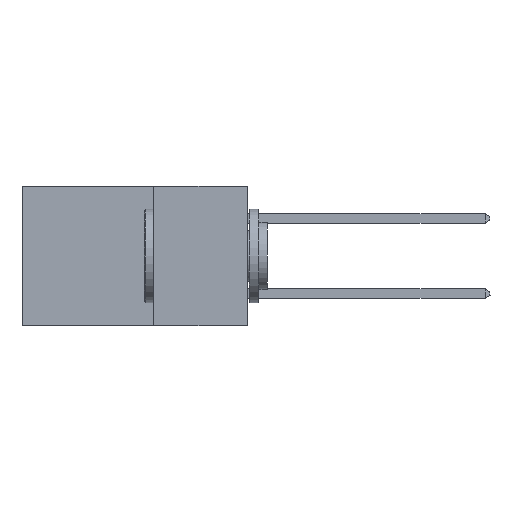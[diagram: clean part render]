
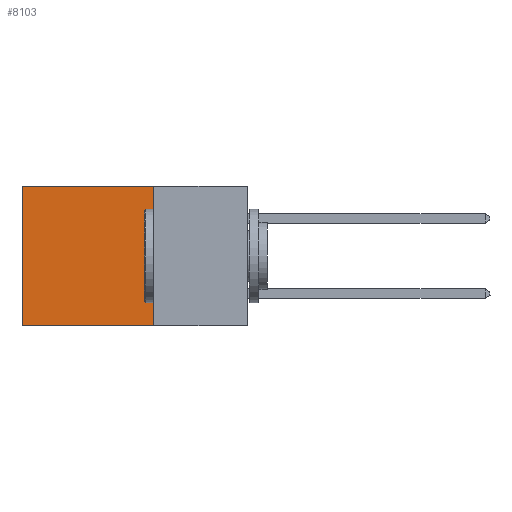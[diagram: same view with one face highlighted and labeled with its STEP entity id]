
A CAD part, left-side view. The second image highlights one B-rep face of the part: STEP entity #8103.
In plain terms, the highlighted planar face has unit normal (-1, 0, 0).
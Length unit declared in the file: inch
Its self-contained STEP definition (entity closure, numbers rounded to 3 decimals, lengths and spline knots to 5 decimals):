
#740 = VECTOR ( 'NONE', #15218, 39.37008 ) ;
#945 = LINE ( 'NONE', #4825, #740 ) ;
#960 = VERTEX_POINT ( 'NONE', #6674 ) ;
#1277 = LINE ( 'NONE', #10558, #10945 ) ;
#1367 = VERTEX_POINT ( 'NONE', #9649 ) ;
#1823 = CARTESIAN_POINT ( 'NONE',  ( 0.298, 0.25, 0. ) ) ;
#2477 = ORIENTED_EDGE ( 'NONE', *, *, #14363, .T. ) ;
#2816 = CARTESIAN_POINT ( 'NONE',  ( 0.298, 0.25, 0. ) ) ;
#3013 = DIRECTION ( 'NONE',  ( 0., 0., -1. ) ) ;
#3215 = DIRECTION ( 'NONE',  ( 1., 0., 0. ) ) ;
#4326 = PLANE ( 'NONE',  #15143 ) ;
#4535 = LINE ( 'NONE', #2816, #12040 ) ;
#4563 = EDGE_LOOP ( 'NONE', ( #7188, #13130, #11146, #2477 ) ) ;
#4825 = CARTESIAN_POINT ( 'NONE',  ( 0.298, 0.25, 0. ) ) ;
#6282 = CARTESIAN_POINT ( 'NONE',  ( 0.298, 0.6, 0. ) ) ;
#6674 = CARTESIAN_POINT ( 'NONE',  ( 0.298, 0.25, -0.37 ) ) ;
#7188 = ORIENTED_EDGE ( 'NONE', *, *, #11415, .T. ) ;
#7447 = VERTEX_POINT ( 'NONE', #6282 ) ;
#7577 = LINE ( 'NONE', #12801, #8155 ) ;
#8010 = DIRECTION ( 'NONE',  ( 0., 0., -1. ) ) ;
#8103 = ADVANCED_FACE ( 'NONE', ( #14569 ), #4326, .F. ) ;
#8155 = VECTOR ( 'NONE', #9005, 39.37008 ) ;
#9005 = DIRECTION ( 'NONE',  ( 0., 1., 0. ) ) ;
#9268 = EDGE_CURVE ( 'NONE', #960, #1367, #7577, .T. ) ;
#9649 = CARTESIAN_POINT ( 'NONE',  ( 0.298, 0.6, -0.37 ) ) ;
#10558 = CARTESIAN_POINT ( 'NONE',  ( 0.298, 0.6, 0. ) ) ;
#10945 = VECTOR ( 'NONE', #3013, 39.37008 ) ;
#11146 = ORIENTED_EDGE ( 'NONE', *, *, #13803, .F. ) ;
#11415 = EDGE_CURVE ( 'NONE', #7447, #1367, #1277, .T. ) ;
#11542 = VERTEX_POINT ( 'NONE', #14204 ) ;
#12040 = VECTOR ( 'NONE', #8010, 39.37008 ) ;
#12801 = CARTESIAN_POINT ( 'NONE',  ( 0.298, 0.25, -0.37 ) ) ;
#13130 = ORIENTED_EDGE ( 'NONE', *, *, #9268, .F. ) ;
#13803 = EDGE_CURVE ( 'NONE', #11542, #960, #4535, .T. ) ;
#14204 = CARTESIAN_POINT ( 'NONE',  ( 0.298, 0.25, 0. ) ) ;
#14363 = EDGE_CURVE ( 'NONE', #11542, #7447, #945, .T. ) ;
#14569 = FACE_OUTER_BOUND ( 'NONE', #4563, .T. ) ;
#15143 = AXIS2_PLACEMENT_3D ( 'NONE', #1823, #3215, #15890 ) ;
#15218 = DIRECTION ( 'NONE',  ( 0., 1., 0. ) ) ;
#15890 = DIRECTION ( 'NONE',  ( 0., 0., -1. ) ) ;
